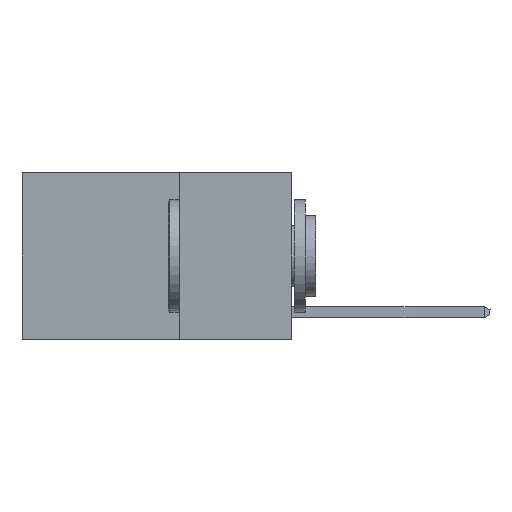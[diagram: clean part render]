
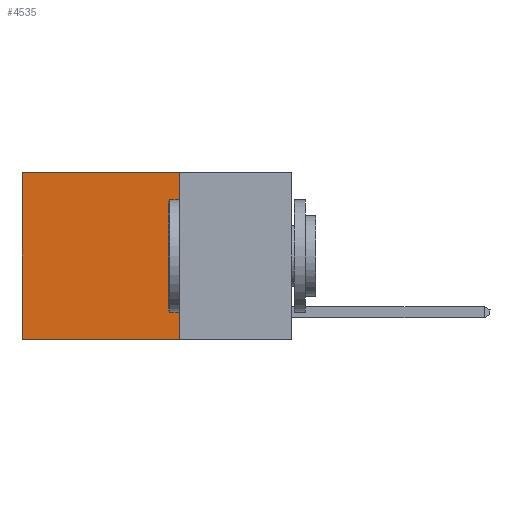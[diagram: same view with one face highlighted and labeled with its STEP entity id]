
A CAD part, left-side view. The second image highlights one B-rep face of the part: STEP entity #4535.
In plain terms, the highlighted planar face has unit normal (-1, 0, 0).
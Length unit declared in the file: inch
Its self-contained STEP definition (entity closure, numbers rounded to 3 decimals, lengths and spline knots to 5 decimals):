
#76 = FACE_OUTER_BOUND ( 'NONE', #3858, .T. ) ;
#526 = EDGE_CURVE ( 'NONE', #15673, #2045, #2729, .T. ) ;
#1410 = AXIS2_PLACEMENT_3D ( 'NONE', #17865, #16491, #5186 ) ;
#2045 = VERTEX_POINT ( 'NONE', #6655 ) ;
#2712 = CARTESIAN_POINT ( 'NONE',  ( 0.2625, 0.25, -0.37 ) ) ;
#2729 = LINE ( 'NONE', #2913, #2946 ) ;
#2913 = CARTESIAN_POINT ( 'NONE',  ( 0.2625, 0.6, 0. ) ) ;
#2946 = VECTOR ( 'NONE', #15771, 39.37008 ) ;
#3238 = CARTESIAN_POINT ( 'NONE',  ( 0.2625, 0.25, -0.37 ) ) ;
#3570 = PLANE ( 'NONE',  #1410 ) ;
#3858 = EDGE_LOOP ( 'NONE', ( #7874, #11494, #14710, #17214 ) ) ;
#4535 = ADVANCED_FACE ( 'NONE', ( #76 ), #3570, .F. ) ;
#4875 = LINE ( 'NONE', #18212, #6425 ) ;
#5186 = DIRECTION ( 'NONE',  ( 0., 0., -1. ) ) ;
#5300 = EDGE_CURVE ( 'NONE', #11794, #13716, #4875, .T. ) ;
#5647 = EDGE_CURVE ( 'NONE', #11794, #15673, #12620, .T. ) ;
#6103 = DIRECTION ( 'NONE',  ( 0., 0., -1. ) ) ;
#6425 = VECTOR ( 'NONE', #6103, 39.37008 ) ;
#6655 = CARTESIAN_POINT ( 'NONE',  ( 0.2625, 0.6, -0.37 ) ) ;
#7552 = DIRECTION ( 'NONE',  ( 0., 1., 0. ) ) ;
#7874 = ORIENTED_EDGE ( 'NONE', *, *, #526, .T. ) ;
#8654 = LINE ( 'NONE', #2712, #16833 ) ;
#8789 = CARTESIAN_POINT ( 'NONE',  ( 0.2625, 0.25, 0. ) ) ;
#10847 = EDGE_CURVE ( 'NONE', #13716, #2045, #8654, .T. ) ;
#11323 = DIRECTION ( 'NONE',  ( 0., 1., 0. ) ) ;
#11494 = ORIENTED_EDGE ( 'NONE', *, *, #10847, .F. ) ;
#11543 = VECTOR ( 'NONE', #7552, 39.37008 ) ;
#11601 = CARTESIAN_POINT ( 'NONE',  ( 0.2625, 0.6, 0. ) ) ;
#11794 = VERTEX_POINT ( 'NONE', #8789 ) ;
#12620 = LINE ( 'NONE', #17380, #11543 ) ;
#13716 = VERTEX_POINT ( 'NONE', #3238 ) ;
#14710 = ORIENTED_EDGE ( 'NONE', *, *, #5300, .F. ) ;
#15673 = VERTEX_POINT ( 'NONE', #11601 ) ;
#15771 = DIRECTION ( 'NONE',  ( 0., 0., -1. ) ) ;
#16491 = DIRECTION ( 'NONE',  ( 1., 0., 0. ) ) ;
#16833 = VECTOR ( 'NONE', #11323, 39.37008 ) ;
#17214 = ORIENTED_EDGE ( 'NONE', *, *, #5647, .T. ) ;
#17380 = CARTESIAN_POINT ( 'NONE',  ( 0.2625, 0.25, 0. ) ) ;
#17865 = CARTESIAN_POINT ( 'NONE',  ( 0.2625, 0.25, 0. ) ) ;
#18212 = CARTESIAN_POINT ( 'NONE',  ( 0.2625, 0.25, 0. ) ) ;
